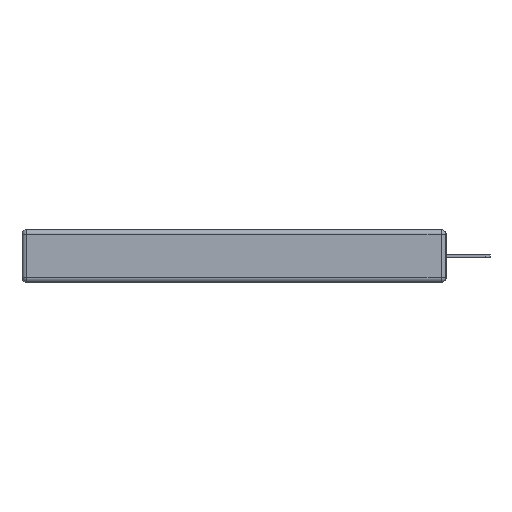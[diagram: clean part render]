
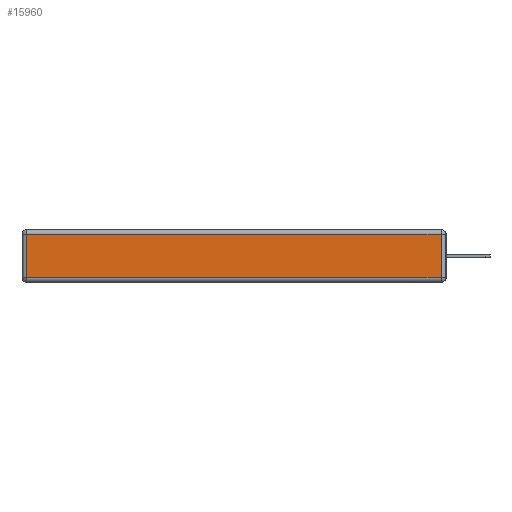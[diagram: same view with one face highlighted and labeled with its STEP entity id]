
A CAD part, left-side view. The second image highlights one B-rep face of the part: STEP entity #15960.
In plain terms, the highlighted planar face has unit normal (-1, 0, 0).
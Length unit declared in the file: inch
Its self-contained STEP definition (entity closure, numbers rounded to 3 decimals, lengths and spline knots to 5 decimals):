
#1045 = ORIENTED_EDGE ( 'NONE', *, *, #5627, .T. ) ;
#1214 = CARTESIAN_POINT ( 'NONE',  ( 0., 0.03, -0.03 ) ) ;
#1389 = DIRECTION ( 'NONE',  ( 0., -1., 0. ) ) ;
#2156 = EDGE_CURVE ( 'NONE', #12332, #6586, #9293, .T. ) ;
#3174 = EDGE_LOOP ( 'NONE', ( #14943, #5289, #8046, #1045 ) ) ;
#4403 = VERTEX_POINT ( 'NONE', #7612 ) ;
#4404 = VECTOR ( 'NONE', #12698, 39.37008 ) ;
#4492 = LINE ( 'NONE', #8504, #4404 ) ;
#5133 = AXIS2_PLACEMENT_3D ( 'NONE', #15067, #12541, #15236 ) ;
#5289 = ORIENTED_EDGE ( 'NONE', *, *, #2156, .T. ) ;
#5475 = VERTEX_POINT ( 'NONE', #12351 ) ;
#5627 = EDGE_CURVE ( 'NONE', #5475, #4403, #4492, .T. ) ;
#6475 = VECTOR ( 'NONE', #11791, 39.37008 ) ;
#6586 = VERTEX_POINT ( 'NONE', #1214 ) ;
#7214 = FACE_OUTER_BOUND ( 'NONE', #3174, .T. ) ;
#7612 = CARTESIAN_POINT ( 'NONE',  ( 0., 2.72, -0.313 ) ) ;
#7720 = CARTESIAN_POINT ( 'NONE',  ( 0., 0.03, -0.343 ) ) ;
#7875 = CARTESIAN_POINT ( 'NONE',  ( 0., 2.75, -0.03 ) ) ;
#8046 = ORIENTED_EDGE ( 'NONE', *, *, #14420, .T. ) ;
#8181 = CARTESIAN_POINT ( 'NONE',  ( 0., 0., -0.313 ) ) ;
#8504 = CARTESIAN_POINT ( 'NONE',  ( 0., 2.72, -0.343 ) ) ;
#9180 = LINE ( 'NONE', #7875, #6475 ) ;
#9226 = VECTOR ( 'NONE', #1389, 39.37008 ) ;
#9293 = LINE ( 'NONE', #7720, #10858 ) ;
#9911 = PLANE ( 'NONE',  #5133 ) ;
#10771 = LINE ( 'NONE', #8181, #9226 ) ;
#10858 = VECTOR ( 'NONE', #14428, 39.37008 ) ;
#11791 = DIRECTION ( 'NONE',  ( 0., 1., 0. ) ) ;
#12173 = CARTESIAN_POINT ( 'NONE',  ( 0., 0.03, -0.313 ) ) ;
#12332 = VERTEX_POINT ( 'NONE', #12173 ) ;
#12351 = CARTESIAN_POINT ( 'NONE',  ( 0., 2.72, -0.03 ) ) ;
#12541 = DIRECTION ( 'NONE',  ( -1., 0., 0. ) ) ;
#12698 = DIRECTION ( 'NONE',  ( 0., 0., -1. ) ) ;
#14420 = EDGE_CURVE ( 'NONE', #6586, #5475, #9180, .T. ) ;
#14428 = DIRECTION ( 'NONE',  ( 0., 0., 1. ) ) ;
#14943 = ORIENTED_EDGE ( 'NONE', *, *, #16983, .T. ) ;
#15067 = CARTESIAN_POINT ( 'NONE',  ( 0., 0., -0.343 ) ) ;
#15236 = DIRECTION ( 'NONE',  ( 0., 0., 1. ) ) ;
#15960 = ADVANCED_FACE ( 'NONE', ( #7214 ), #9911, .T. ) ;
#16983 = EDGE_CURVE ( 'NONE', #4403, #12332, #10771, .T. ) ;
